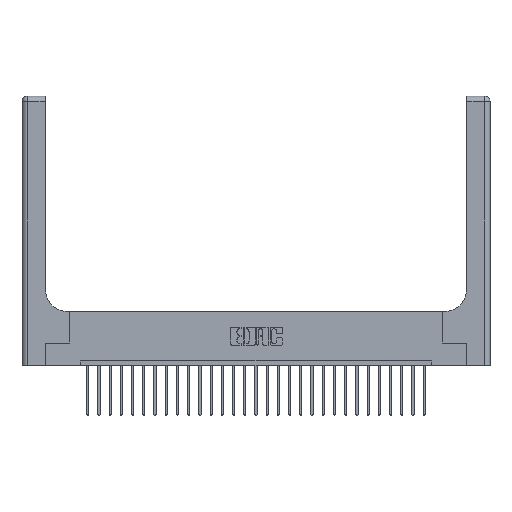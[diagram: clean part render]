
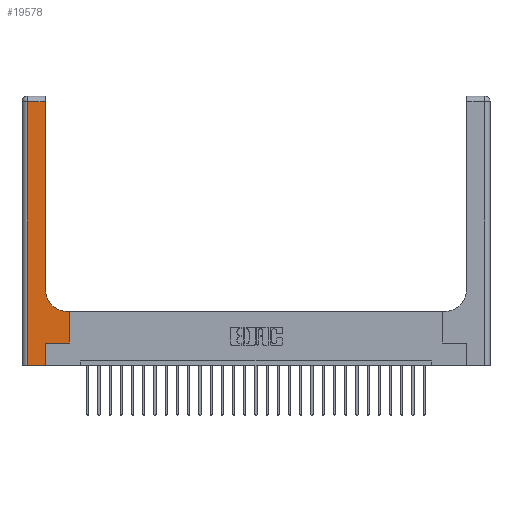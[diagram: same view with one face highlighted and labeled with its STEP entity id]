
A CAD part, top view. The second image highlights one B-rep face of the part: STEP entity #19578.
In plain terms, the highlighted planar face has unit normal (0, 0, 1).
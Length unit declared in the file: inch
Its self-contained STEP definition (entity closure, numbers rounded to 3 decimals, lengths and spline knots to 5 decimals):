
#42 = CARTESIAN_POINT ( 'NONE',  ( 0.265, 0., 0.37 ) ) ;
#210 = EDGE_CURVE ( 'NONE', #10316, #25746, #23793, .T. ) ;
#539 = CARTESIAN_POINT ( 'NONE',  ( 0., 2.94, 0.37 ) ) ;
#922 = EDGE_CURVE ( 'NONE', #12246, #10834, #6190, .T. ) ;
#1097 = CARTESIAN_POINT ( 'NONE',  ( 0.26, 3., 0.37 ) ) ;
#1101 = CARTESIAN_POINT ( 'NONE',  ( 0.265, 0., 0.37 ) ) ;
#1192 = LINE ( 'NONE', #22004, #12185 ) ;
#1507 = EDGE_LOOP ( 'NONE', ( #18614, #12582, #12945, #21543, #2048, #18545, #7823, #9063, #8682 ) ) ;
#1571 = LINE ( 'NONE', #23220, #13506 ) ;
#2045 = CARTESIAN_POINT ( 'NONE',  ( 0.265, 0.25, 0.37 ) ) ;
#2048 = ORIENTED_EDGE ( 'NONE', *, *, #19551, .T. ) ;
#2074 = CARTESIAN_POINT ( 'NONE',  ( 0.265, 0.25, 0.37 ) ) ;
#3181 = VECTOR ( 'NONE', #6842, 39.37008 ) ;
#3403 = DIRECTION ( 'NONE',  ( -1., 0., 0. ) ) ;
#3805 = VECTOR ( 'NONE', #23864, 39.37008 ) ;
#4343 = VERTEX_POINT ( 'NONE', #1101 ) ;
#4376 = EDGE_CURVE ( 'NONE', #22639, #10078, #1192, .T. ) ;
#4624 = LINE ( 'NONE', #20920, #10231 ) ;
#5028 = DIRECTION ( 'NONE',  ( 0., 0., -1. ) ) ;
#5926 = VECTOR ( 'NONE', #11762, 39.37008 ) ;
#6190 = CIRCLE ( 'NONE', #16603, 0.25 ) ;
#6292 = FACE_OUTER_BOUND ( 'NONE', #1507, .T. ) ;
#6842 = DIRECTION ( 'NONE',  ( 0., 1., 0. ) ) ;
#6987 = DIRECTION ( 'NONE',  ( 1., 0., 0. ) ) ;
#7383 = CARTESIAN_POINT ( 'NONE',  ( 0.528, 0.6, 0.37 ) ) ;
#7823 = ORIENTED_EDGE ( 'NONE', *, *, #210, .T. ) ;
#8158 = DIRECTION ( 'NONE',  ( -1., 0., 0. ) ) ;
#8330 = CARTESIAN_POINT ( 'NONE',  ( 0.06, 2.94, 0.37 ) ) ;
#8682 = ORIENTED_EDGE ( 'NONE', *, *, #922, .T. ) ;
#9063 = ORIENTED_EDGE ( 'NONE', *, *, #16177, .T. ) ;
#9270 = EDGE_CURVE ( 'NONE', #10078, #4343, #1571, .T. ) ;
#9662 = CARTESIAN_POINT ( 'NONE',  ( 0.528, 0.25, 0.37 ) ) ;
#9922 = VECTOR ( 'NONE', #3403, 39.37008 ) ;
#10011 = VERTEX_POINT ( 'NONE', #15184 ) ;
#10078 = VERTEX_POINT ( 'NONE', #13319 ) ;
#10231 = VECTOR ( 'NONE', #21180, 39.37008 ) ;
#10316 = VERTEX_POINT ( 'NONE', #14668 ) ;
#10449 = PLANE ( 'NONE',  #22240 ) ;
#10834 = VERTEX_POINT ( 'NONE', #18332 ) ;
#10992 = LINE ( 'NONE', #42, #21658 ) ;
#11762 = DIRECTION ( 'NONE',  ( 0., 1., 0. ) ) ;
#12123 = DIRECTION ( 'NONE',  ( 0., -1., 0. ) ) ;
#12185 = VECTOR ( 'NONE', #12123, 39.37008 ) ;
#12246 = VERTEX_POINT ( 'NONE', #24614 ) ;
#12291 = LINE ( 'NONE', #2074, #3805 ) ;
#12582 = ORIENTED_EDGE ( 'NONE', *, *, #22031, .T. ) ;
#12945 = ORIENTED_EDGE ( 'NONE', *, *, #4376, .T. ) ;
#13319 = CARTESIAN_POINT ( 'NONE',  ( 0.06, 0., 0.37 ) ) ;
#13506 = VECTOR ( 'NONE', #17359, 39.37008 ) ;
#14067 = DIRECTION ( 'NONE',  ( 0., 1., 0. ) ) ;
#14668 = CARTESIAN_POINT ( 'NONE',  ( 0.528, 0.25, 0.37 ) ) ;
#15184 = CARTESIAN_POINT ( 'NONE',  ( 0.26, 2.94, 0.37 ) ) ;
#15783 = LINE ( 'NONE', #1097, #3181 ) ;
#16177 = EDGE_CURVE ( 'NONE', #25746, #12246, #4624, .T. ) ;
#16603 = AXIS2_PLACEMENT_3D ( 'NONE', #24982, #5028, #6987 ) ;
#17359 = DIRECTION ( 'NONE',  ( 1., 0., 0. ) ) ;
#18112 = LINE ( 'NONE', #539, #9922 ) ;
#18332 = CARTESIAN_POINT ( 'NONE',  ( 0.26, 0.85, 0.37 ) ) ;
#18545 = ORIENTED_EDGE ( 'NONE', *, *, #25002, .T. ) ;
#18614 = ORIENTED_EDGE ( 'NONE', *, *, #19347, .T. ) ;
#19347 = EDGE_CURVE ( 'NONE', #10834, #10011, #15783, .T. ) ;
#19551 = EDGE_CURVE ( 'NONE', #4343, #20945, #10992, .T. ) ;
#19578 = ADVANCED_FACE ( 'NONE', ( #6292 ), #10449, .F. ) ;
#20190 = CARTESIAN_POINT ( 'NONE',  ( 0., 3., 0.37 ) ) ;
#20920 = CARTESIAN_POINT ( 'NONE',  ( 0.26, 0.6, 0.37 ) ) ;
#20945 = VERTEX_POINT ( 'NONE', #2045 ) ;
#21180 = DIRECTION ( 'NONE',  ( -1., 0., 0. ) ) ;
#21543 = ORIENTED_EDGE ( 'NONE', *, *, #9270, .T. ) ;
#21658 = VECTOR ( 'NONE', #14067, 39.37008 ) ;
#22004 = CARTESIAN_POINT ( 'NONE',  ( 0.06, 3., 0.37 ) ) ;
#22031 = EDGE_CURVE ( 'NONE', #10011, #22639, #18112, .T. ) ;
#22240 = AXIS2_PLACEMENT_3D ( 'NONE', #20190, #24469, #8158 ) ;
#22639 = VERTEX_POINT ( 'NONE', #8330 ) ;
#23220 = CARTESIAN_POINT ( 'NONE',  ( 0., 0., 0.37 ) ) ;
#23793 = LINE ( 'NONE', #9662, #5926 ) ;
#23864 = DIRECTION ( 'NONE',  ( 1., 0., 0. ) ) ;
#24469 = DIRECTION ( 'NONE',  ( 0., 0., -1. ) ) ;
#24614 = CARTESIAN_POINT ( 'NONE',  ( 0.51, 0.6, 0.37 ) ) ;
#24982 = CARTESIAN_POINT ( 'NONE',  ( 0.51, 0.85, 0.37 ) ) ;
#25002 = EDGE_CURVE ( 'NONE', #20945, #10316, #12291, .T. ) ;
#25746 = VERTEX_POINT ( 'NONE', #7383 ) ;
